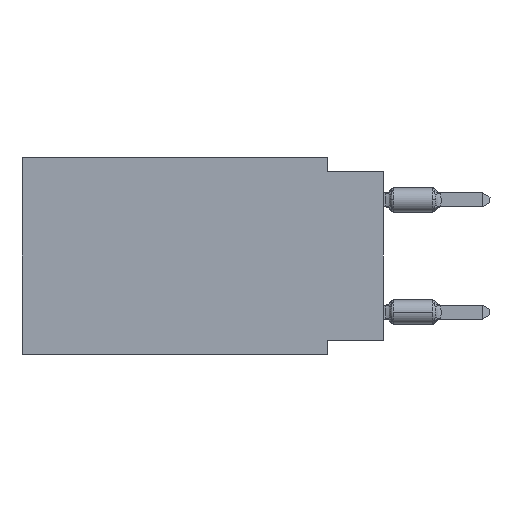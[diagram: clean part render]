
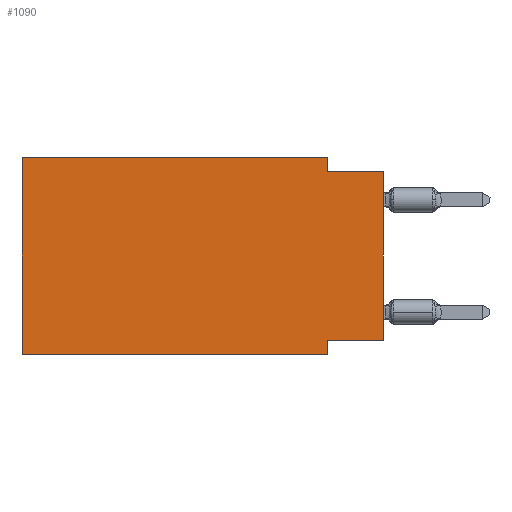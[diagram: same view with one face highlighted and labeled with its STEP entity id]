
A CAD part, left-side view. The second image highlights one B-rep face of the part: STEP entity #1090.
In plain terms, the highlighted planar face has unit normal (-1, 0, 0).
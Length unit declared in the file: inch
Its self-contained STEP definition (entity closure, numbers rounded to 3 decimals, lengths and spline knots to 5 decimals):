
#494 = CARTESIAN_POINT ( 'NONE',  ( 0., 0., -0.025 ) ) ;
#710 = CARTESIAN_POINT ( 'NONE',  ( 0., 0.1, 0. ) ) ;
#760 = CARTESIAN_POINT ( 'NONE',  ( 0., 0.645, -0.35 ) ) ;
#782 = VECTOR ( 'NONE', #794, 39.37008 ) ;
#794 = DIRECTION ( 'NONE',  ( 0., 0., -1. ) ) ;
#1002 = DIRECTION ( 'NONE',  ( 0., 0., -1. ) ) ;
#1090 = ADVANCED_FACE ( 'NONE', ( #4561 ), #6024, .F. ) ;
#1710 = VECTOR ( 'NONE', #16598, 39.37008 ) ;
#3145 = LINE ( 'NONE', #14906, #7729 ) ;
#3211 = EDGE_CURVE ( 'NONE', #6092, #5383, #13917, .T. ) ;
#3549 = EDGE_LOOP ( 'NONE', ( #16442, #7760, #6895, #14568, #14727, #4550, #9011, #15809 ) ) ;
#4550 = ORIENTED_EDGE ( 'NONE', *, *, #3211, .T. ) ;
#4561 = FACE_OUTER_BOUND ( 'NONE', #3549, .T. ) ;
#4777 = CARTESIAN_POINT ( 'NONE',  ( 0., 0.1, 0. ) ) ;
#5202 = CARTESIAN_POINT ( 'NONE',  ( 0., 0.1, -0.325 ) ) ;
#5323 = VERTEX_POINT ( 'NONE', #4777 ) ;
#5381 = EDGE_CURVE ( 'NONE', #5323, #13498, #7195, .T. ) ;
#5383 = VERTEX_POINT ( 'NONE', #8508 ) ;
#5397 = EDGE_CURVE ( 'NONE', #6092, #10630, #13869, .T. ) ;
#6024 = PLANE ( 'NONE',  #12516 ) ;
#6042 = CARTESIAN_POINT ( 'NONE',  ( 0., 0.645, 0. ) ) ;
#6092 = VERTEX_POINT ( 'NONE', #6878 ) ;
#6106 = DIRECTION ( 'NONE',  ( 1., 0., 0. ) ) ;
#6746 = CARTESIAN_POINT ( 'NONE',  ( 0., 0., -0.325 ) ) ;
#6878 = CARTESIAN_POINT ( 'NONE',  ( 0., 0.645, -0.35 ) ) ;
#6895 = ORIENTED_EDGE ( 'NONE', *, *, #5381, .F. ) ;
#7136 = VECTOR ( 'NONE', #16384, 39.37008 ) ;
#7195 = LINE ( 'NONE', #710, #782 ) ;
#7497 = VECTOR ( 'NONE', #13343, 39.37008 ) ;
#7621 = VERTEX_POINT ( 'NONE', #494 ) ;
#7729 = VECTOR ( 'NONE', #13689, 39.37008 ) ;
#7760 = ORIENTED_EDGE ( 'NONE', *, *, #8326, .F. ) ;
#8326 = EDGE_CURVE ( 'NONE', #13498, #7621, #14655, .T. ) ;
#8508 = CARTESIAN_POINT ( 'NONE',  ( 0., 0.1, -0.35 ) ) ;
#8781 = EDGE_CURVE ( 'NONE', #10630, #5323, #16256, .T. ) ;
#9011 = ORIENTED_EDGE ( 'NONE', *, *, #15653, .F. ) ;
#9658 = VERTEX_POINT ( 'NONE', #14115 ) ;
#9799 = CARTESIAN_POINT ( 'NONE',  ( 0., 0.1, -0.025 ) ) ;
#10630 = VERTEX_POINT ( 'NONE', #14202 ) ;
#11055 = DIRECTION ( 'NONE',  ( 0., -1., 0. ) ) ;
#11092 = CARTESIAN_POINT ( 'NONE',  ( 0., 0.645, 0. ) ) ;
#11381 = CARTESIAN_POINT ( 'NONE',  ( 0., 0.645, 0. ) ) ;
#12128 = EDGE_CURVE ( 'NONE', #9658, #15113, #14626, .T. ) ;
#12337 = DIRECTION ( 'NONE',  ( 0., 0., -1. ) ) ;
#12516 = AXIS2_PLACEMENT_3D ( 'NONE', #11381, #6106, #1002 ) ;
#12989 = VECTOR ( 'NONE', #12337, 39.37008 ) ;
#13343 = DIRECTION ( 'NONE',  ( 0., -1., 0. ) ) ;
#13498 = VERTEX_POINT ( 'NONE', #9799 ) ;
#13596 = VECTOR ( 'NONE', #11055, 39.37008 ) ;
#13689 = DIRECTION ( 'NONE',  ( 0., 0., 1. ) ) ;
#13869 = LINE ( 'NONE', #11092, #7136 ) ;
#13917 = LINE ( 'NONE', #760, #1710 ) ;
#14115 = CARTESIAN_POINT ( 'NONE',  ( 0., 0., -0.325 ) ) ;
#14135 = DIRECTION ( 'NONE',  ( 0., 1., 0. ) ) ;
#14202 = CARTESIAN_POINT ( 'NONE',  ( 0., 0.645, 0. ) ) ;
#14483 = CARTESIAN_POINT ( 'NONE',  ( 0., 0., -0.025 ) ) ;
#14568 = ORIENTED_EDGE ( 'NONE', *, *, #8781, .F. ) ;
#14626 = LINE ( 'NONE', #6746, #16443 ) ;
#14655 = LINE ( 'NONE', #14483, #7497 ) ;
#14727 = ORIENTED_EDGE ( 'NONE', *, *, #5397, .F. ) ;
#14788 = EDGE_CURVE ( 'NONE', #9658, #7621, #3145, .T. ) ;
#14906 = CARTESIAN_POINT ( 'NONE',  ( 0., 0., 0. ) ) ;
#14951 = LINE ( 'NONE', #16336, #12989 ) ;
#15113 = VERTEX_POINT ( 'NONE', #5202 ) ;
#15653 = EDGE_CURVE ( 'NONE', #15113, #5383, #14951, .T. ) ;
#15809 = ORIENTED_EDGE ( 'NONE', *, *, #12128, .F. ) ;
#16256 = LINE ( 'NONE', #6042, #13596 ) ;
#16336 = CARTESIAN_POINT ( 'NONE',  ( 0., 0.1, -0.35 ) ) ;
#16384 = DIRECTION ( 'NONE',  ( 0., 0., 1. ) ) ;
#16442 = ORIENTED_EDGE ( 'NONE', *, *, #14788, .T. ) ;
#16443 = VECTOR ( 'NONE', #14135, 39.37008 ) ;
#16598 = DIRECTION ( 'NONE',  ( 0., -1., 0. ) ) ;
